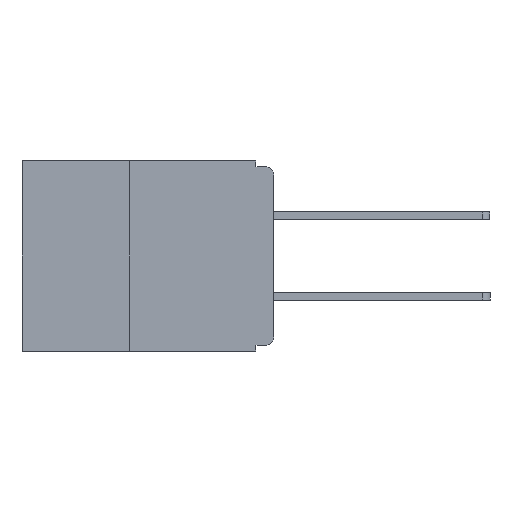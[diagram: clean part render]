
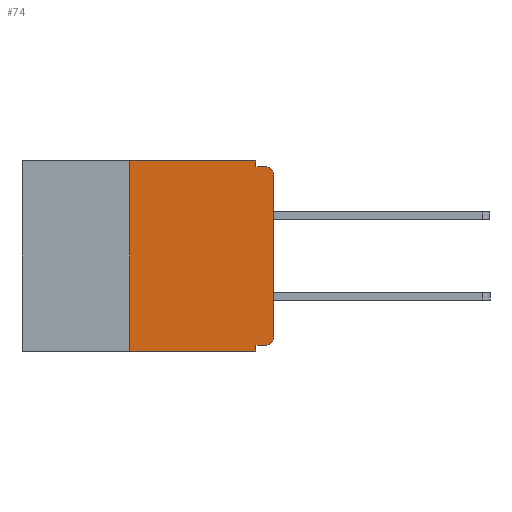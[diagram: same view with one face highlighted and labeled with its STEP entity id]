
A CAD part, left-side view. The second image highlights one B-rep face of the part: STEP entity #74.
In plain terms, the highlighted planar face has unit normal (-1, 0, 0).
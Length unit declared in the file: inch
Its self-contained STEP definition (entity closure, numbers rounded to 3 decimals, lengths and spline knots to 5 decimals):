
#57 = VECTOR ( 'NONE', #10425, 39.37008 ) ;
#74 = ADVANCED_FACE ( 'NONE', ( #10110 ), #1163, .F. ) ;
#289 = EDGE_CURVE ( 'NONE', #2214, #13374, #10299, .T. ) ;
#431 = AXIS2_PLACEMENT_3D ( 'NONE', #12259, #4638, #13493 ) ;
#493 = VERTEX_POINT ( 'NONE', #7901 ) ;
#509 = ORIENTED_EDGE ( 'NONE', *, *, #6179, .T. ) ;
#736 = CARTESIAN_POINT ( 'NONE',  ( 0., 0.25, -0.33 ) ) ;
#762 = CARTESIAN_POINT ( 'NONE',  ( 0., 0., -0.01 ) ) ;
#903 = EDGE_CURVE ( 'NONE', #10266, #12722, #8274, .T. ) ;
#1043 = VECTOR ( 'NONE', #4694, 39.37008 ) ;
#1163 = PLANE ( 'NONE',  #16255 ) ;
#1213 = VERTEX_POINT ( 'NONE', #10334 ) ;
#1406 = CARTESIAN_POINT ( 'NONE',  ( 0., 0.437, -0.33 ) ) ;
#1597 = DIRECTION ( 'NONE',  ( 0., -1., 0. ) ) ;
#1661 = CARTESIAN_POINT ( 'NONE',  ( 0., 0., -0.305 ) ) ;
#1805 = VECTOR ( 'NONE', #3045, 39.37008 ) ;
#2214 = VERTEX_POINT ( 'NONE', #1661 ) ;
#2232 = ORIENTED_EDGE ( 'NONE', *, *, #16269, .F. ) ;
#2640 = EDGE_CURVE ( 'NONE', #493, #4522, #9830, .T. ) ;
#2965 = EDGE_CURVE ( 'NONE', #1213, #4021, #11642, .T. ) ;
#3013 = CARTESIAN_POINT ( 'NONE',  ( 0., 0.015, -0.01 ) ) ;
#3045 = DIRECTION ( 'NONE',  ( 0., 0., -1. ) ) ;
#3100 = CARTESIAN_POINT ( 'NONE',  ( 0., 0.031, -0.33 ) ) ;
#3349 = CARTESIAN_POINT ( 'NONE',  ( 0., 0.25, 0. ) ) ;
#3761 = ORIENTED_EDGE ( 'NONE', *, *, #289, .T. ) ;
#4021 = VERTEX_POINT ( 'NONE', #11933 ) ;
#4249 = ORIENTED_EDGE ( 'NONE', *, *, #13315, .T. ) ;
#4522 = VERTEX_POINT ( 'NONE', #16293 ) ;
#4534 = CARTESIAN_POINT ( 'NONE',  ( 0., 0.25, -0.33 ) ) ;
#4638 = DIRECTION ( 'NONE',  ( -1., 0., 0. ) ) ;
#4694 = DIRECTION ( 'NONE',  ( 0., 0., 1. ) ) ;
#4985 = LINE ( 'NONE', #9578, #14670 ) ;
#5931 = DIRECTION ( 'NONE',  ( 0., 0., -1. ) ) ;
#6179 = EDGE_CURVE ( 'NONE', #13374, #9491, #7386, .T. ) ;
#6762 = EDGE_CURVE ( 'NONE', #12722, #493, #4985, .T. ) ;
#7253 = EDGE_CURVE ( 'NONE', #10266, #4021, #14653, .T. ) ;
#7386 = CIRCLE ( 'NONE', #13533, 0.015 ) ;
#7449 = ORIENTED_EDGE ( 'NONE', *, *, #6762, .F. ) ;
#7731 = ORIENTED_EDGE ( 'NONE', *, *, #903, .F. ) ;
#7901 = CARTESIAN_POINT ( 'NONE',  ( 0., 0.031, 0. ) ) ;
#8274 = LINE ( 'NONE', #736, #1043 ) ;
#8589 = CARTESIAN_POINT ( 'NONE',  ( 0., 0., -0.32 ) ) ;
#9004 = EDGE_CURVE ( 'NONE', #4522, #9491, #12862, .T. ) ;
#9017 = CIRCLE ( 'NONE', #431, 0.015 ) ;
#9022 = CARTESIAN_POINT ( 'NONE',  ( 0., 0., 0. ) ) ;
#9425 = VECTOR ( 'NONE', #14726, 39.37008 ) ;
#9491 = VERTEX_POINT ( 'NONE', #3013 ) ;
#9504 = DIRECTION ( 'NONE',  ( 0., -1., 0. ) ) ;
#9514 = VECTOR ( 'NONE', #12308, 39.37008 ) ;
#9578 = CARTESIAN_POINT ( 'NONE',  ( 0., 0.437, 0. ) ) ;
#9702 = VECTOR ( 'NONE', #12357, 39.37008 ) ;
#9830 = LINE ( 'NONE', #12668, #9425 ) ;
#9920 = DIRECTION ( 'NONE',  ( -1., 0., 0. ) ) ;
#10029 = CARTESIAN_POINT ( 'NONE',  ( 0., 0.015, -0.025 ) ) ;
#10110 = FACE_OUTER_BOUND ( 'NONE', #11846, .T. ) ;
#10266 = VERTEX_POINT ( 'NONE', #4534 ) ;
#10299 = LINE ( 'NONE', #9022, #57 ) ;
#10314 = ORIENTED_EDGE ( 'NONE', *, *, #2965, .F. ) ;
#10334 = CARTESIAN_POINT ( 'NONE',  ( 0., 0.031, -0.32 ) ) ;
#10425 = DIRECTION ( 'NONE',  ( 0., 0., 1. ) ) ;
#10833 = VERTEX_POINT ( 'NONE', #12114 ) ;
#11124 = CARTESIAN_POINT ( 'NONE',  ( 0., 0., -0.025 ) ) ;
#11642 = LINE ( 'NONE', #3100, #1805 ) ;
#11846 = EDGE_LOOP ( 'NONE', ( #3761, #509, #16338, #14842, #7449, #7731, #12027, #10314, #2232, #4249 ) ) ;
#11933 = CARTESIAN_POINT ( 'NONE',  ( 0., 0.031, -0.33 ) ) ;
#12027 = ORIENTED_EDGE ( 'NONE', *, *, #7253, .T. ) ;
#12114 = CARTESIAN_POINT ( 'NONE',  ( 0., 0.015, -0.32 ) ) ;
#12259 = CARTESIAN_POINT ( 'NONE',  ( 0., 0.015, -0.305 ) ) ;
#12308 = DIRECTION ( 'NONE',  ( 0., -1., 0. ) ) ;
#12357 = DIRECTION ( 'NONE',  ( 0., 1., 0. ) ) ;
#12364 = DIRECTION ( 'NONE',  ( 0., 0., -1. ) ) ;
#12668 = CARTESIAN_POINT ( 'NONE',  ( 0., 0.031, 0. ) ) ;
#12722 = VERTEX_POINT ( 'NONE', #3349 ) ;
#12862 = LINE ( 'NONE', #762, #9514 ) ;
#13315 = EDGE_CURVE ( 'NONE', #10833, #2214, #9017, .T. ) ;
#13372 = DIRECTION ( 'NONE',  ( 1., 0., 0. ) ) ;
#13374 = VERTEX_POINT ( 'NONE', #11124 ) ;
#13493 = DIRECTION ( 'NONE',  ( 0., 0., -1. ) ) ;
#13533 = AXIS2_PLACEMENT_3D ( 'NONE', #10029, #9920, #12364 ) ;
#14272 = VECTOR ( 'NONE', #1597, 39.37008 ) ;
#14653 = LINE ( 'NONE', #1406, #14272 ) ;
#14670 = VECTOR ( 'NONE', #9504, 39.37008 ) ;
#14726 = DIRECTION ( 'NONE',  ( 0., 0., -1. ) ) ;
#14842 = ORIENTED_EDGE ( 'NONE', *, *, #2640, .F. ) ;
#15148 = LINE ( 'NONE', #8589, #9702 ) ;
#16204 = CARTESIAN_POINT ( 'NONE',  ( 0., 0.437, 0. ) ) ;
#16255 = AXIS2_PLACEMENT_3D ( 'NONE', #16204, #13372, #5931 ) ;
#16269 = EDGE_CURVE ( 'NONE', #10833, #1213, #15148, .T. ) ;
#16293 = CARTESIAN_POINT ( 'NONE',  ( 0., 0.031, -0.01 ) ) ;
#16338 = ORIENTED_EDGE ( 'NONE', *, *, #9004, .F. ) ;
